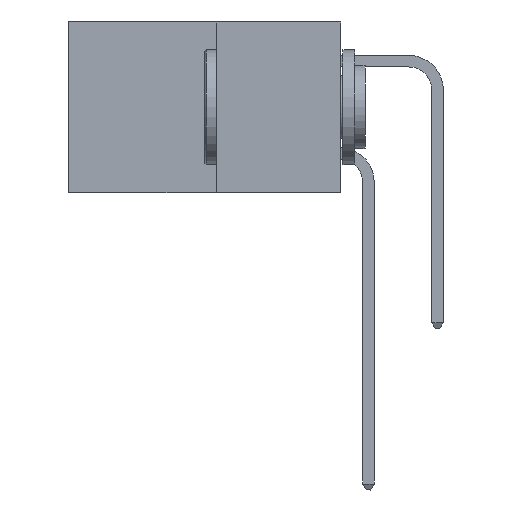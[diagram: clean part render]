
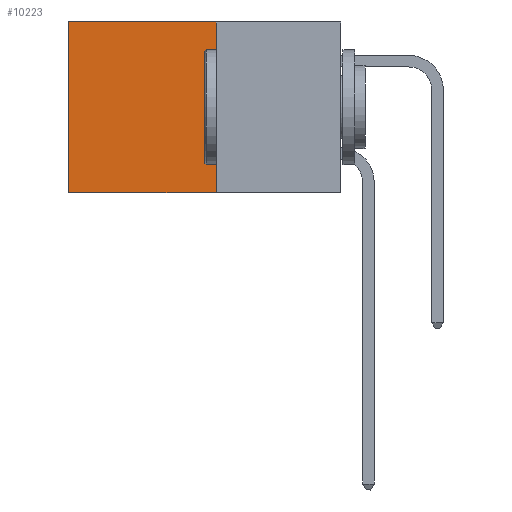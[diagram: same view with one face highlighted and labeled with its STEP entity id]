
A CAD part, left-side view. The second image highlights one B-rep face of the part: STEP entity #10223.
In plain terms, the highlighted planar face has unit normal (-1, 0, 0).
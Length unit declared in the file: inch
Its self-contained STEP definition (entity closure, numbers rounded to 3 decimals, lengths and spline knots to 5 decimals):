
#80 = EDGE_LOOP ( 'NONE', ( #27375, #27104, #31534, #14383 ) ) ;
#878 = CARTESIAN_POINT ( 'NONE',  ( 0.277, 0.59, -0.37 ) ) ;
#1145 = DIRECTION ( 'NONE',  ( 0., 1., 0. ) ) ;
#1466 = LINE ( 'NONE', #1927, #26978 ) ;
#1899 = VECTOR ( 'NONE', #17316, 39.37008 ) ;
#1927 = CARTESIAN_POINT ( 'NONE',  ( 0.277, 0.27, -0.37 ) ) ;
#2661 = LINE ( 'NONE', #29643, #1899 ) ;
#3014 = CARTESIAN_POINT ( 'NONE',  ( 0.277, 0.27, -0.37 ) ) ;
#3125 = DIRECTION ( 'NONE',  ( 1., 0., 0. ) ) ;
#7339 = EDGE_CURVE ( 'NONE', #9950, #15133, #1466, .T. ) ;
#9950 = VERTEX_POINT ( 'NONE', #19340 ) ;
#10223 = ADVANCED_FACE ( 'NONE', ( #22989 ), #25327, .F. ) ;
#10532 = AXIS2_PLACEMENT_3D ( 'NONE', #3014, #3125, #20428 ) ;
#10824 = CARTESIAN_POINT ( 'NONE',  ( 0.277, 0.27, 0. ) ) ;
#10961 = VECTOR ( 'NONE', #14809, 39.37008 ) ;
#11720 = LINE ( 'NONE', #29587, #10961 ) ;
#12260 = EDGE_CURVE ( 'NONE', #19006, #15133, #19619, .T. ) ;
#14383 = ORIENTED_EDGE ( 'NONE', *, *, #27012, .T. ) ;
#14809 = DIRECTION ( 'NONE',  ( 0., 0., -1. ) ) ;
#14926 = CARTESIAN_POINT ( 'NONE',  ( 0.277, 0.59, -0.37 ) ) ;
#15133 = VERTEX_POINT ( 'NONE', #14926 ) ;
#17316 = DIRECTION ( 'NONE',  ( 0., 1., 0. ) ) ;
#19006 = VERTEX_POINT ( 'NONE', #28699 ) ;
#19340 = CARTESIAN_POINT ( 'NONE',  ( 0.277, 0.27, -0.37 ) ) ;
#19619 = LINE ( 'NONE', #878, #31921 ) ;
#20428 = DIRECTION ( 'NONE',  ( 0., 0., -1. ) ) ;
#20534 = EDGE_CURVE ( 'NONE', #25313, #9950, #11720, .T. ) ;
#20678 = DIRECTION ( 'NONE',  ( 0., 0., -1. ) ) ;
#22989 = FACE_OUTER_BOUND ( 'NONE', #80, .T. ) ;
#25313 = VERTEX_POINT ( 'NONE', #10824 ) ;
#25327 = PLANE ( 'NONE',  #10532 ) ;
#26978 = VECTOR ( 'NONE', #1145, 39.37008 ) ;
#27012 = EDGE_CURVE ( 'NONE', #25313, #19006, #2661, .T. ) ;
#27104 = ORIENTED_EDGE ( 'NONE', *, *, #7339, .F. ) ;
#27375 = ORIENTED_EDGE ( 'NONE', *, *, #12260, .T. ) ;
#28699 = CARTESIAN_POINT ( 'NONE',  ( 0.277, 0.59, 0. ) ) ;
#29587 = CARTESIAN_POINT ( 'NONE',  ( 0.277, 0.27, -0.37 ) ) ;
#29643 = CARTESIAN_POINT ( 'NONE',  ( 0.277, 0.27, 0. ) ) ;
#31534 = ORIENTED_EDGE ( 'NONE', *, *, #20534, .F. ) ;
#31921 = VECTOR ( 'NONE', #20678, 39.37008 ) ;
